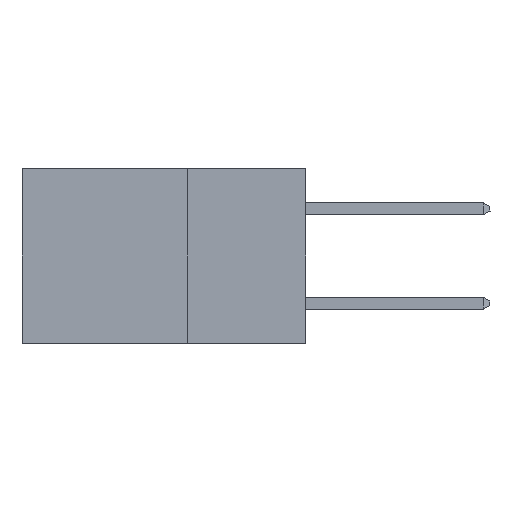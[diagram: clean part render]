
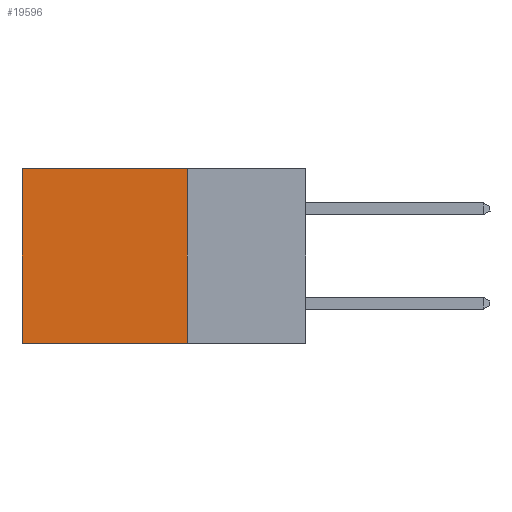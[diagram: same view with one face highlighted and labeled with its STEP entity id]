
A CAD part, left-side view. The second image highlights one B-rep face of the part: STEP entity #19596.
In plain terms, the highlighted planar face has unit normal (-1, 0, 0).
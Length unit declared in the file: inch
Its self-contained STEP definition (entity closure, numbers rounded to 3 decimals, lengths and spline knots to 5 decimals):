
#124 = VECTOR ( 'NONE', #10362, 39.37008 ) ;
#662 = EDGE_CURVE ( 'NONE', #23509, #13252, #12239, .T. ) ;
#1807 = CARTESIAN_POINT ( 'NONE',  ( 0.298, 0.25, -0.37 ) ) ;
#2325 = ORIENTED_EDGE ( 'NONE', *, *, #30814, .F. ) ;
#2909 = CARTESIAN_POINT ( 'NONE',  ( 0.298, 0.6, 0. ) ) ;
#3362 = CARTESIAN_POINT ( 'NONE',  ( 0.298, 0.25, 0. ) ) ;
#3587 = VERTEX_POINT ( 'NONE', #17950 ) ;
#3789 = DIRECTION ( 'NONE',  ( 0., 0., -1. ) ) ;
#4564 = DIRECTION ( 'NONE',  ( 0., 1., 0. ) ) ;
#4789 = DIRECTION ( 'NONE',  ( 0., 0., -1. ) ) ;
#5331 = ORIENTED_EDGE ( 'NONE', *, *, #23557, .T. ) ;
#5477 = VECTOR ( 'NONE', #4564, 39.37008 ) ;
#5871 = LINE ( 'NONE', #1807, #5477 ) ;
#7683 = DIRECTION ( 'NONE',  ( 0., 0., -1. ) ) ;
#7885 = LINE ( 'NONE', #2909, #26384 ) ;
#10362 = DIRECTION ( 'NONE',  ( 0., 1., 0. ) ) ;
#11005 = AXIS2_PLACEMENT_3D ( 'NONE', #16033, #16863, #4789 ) ;
#12239 = LINE ( 'NONE', #3362, #124 ) ;
#12748 = VECTOR ( 'NONE', #3789, 39.37008 ) ;
#13252 = VERTEX_POINT ( 'NONE', #20198 ) ;
#14552 = CARTESIAN_POINT ( 'NONE',  ( 0.298, 0.25, 0. ) ) ;
#15686 = EDGE_CURVE ( 'NONE', #23509, #3587, #18451, .T. ) ;
#16033 = CARTESIAN_POINT ( 'NONE',  ( 0.298, 0.25, 0. ) ) ;
#16215 = ORIENTED_EDGE ( 'NONE', *, *, #662, .T. ) ;
#16863 = DIRECTION ( 'NONE',  ( 1., 0., 0. ) ) ;
#17950 = CARTESIAN_POINT ( 'NONE',  ( 0.298, 0.25, -0.37 ) ) ;
#18451 = LINE ( 'NONE', #18626, #12748 ) ;
#18626 = CARTESIAN_POINT ( 'NONE',  ( 0.298, 0.25, 0. ) ) ;
#18630 = EDGE_LOOP ( 'NONE', ( #5331, #2325, #23736, #16215 ) ) ;
#19596 = ADVANCED_FACE ( 'NONE', ( #24249 ), #30500, .F. ) ;
#20198 = CARTESIAN_POINT ( 'NONE',  ( 0.298, 0.6, 0. ) ) ;
#20224 = VERTEX_POINT ( 'NONE', #26905 ) ;
#23509 = VERTEX_POINT ( 'NONE', #14552 ) ;
#23557 = EDGE_CURVE ( 'NONE', #13252, #20224, #7885, .T. ) ;
#23736 = ORIENTED_EDGE ( 'NONE', *, *, #15686, .F. ) ;
#24249 = FACE_OUTER_BOUND ( 'NONE', #18630, .T. ) ;
#26384 = VECTOR ( 'NONE', #7683, 39.37008 ) ;
#26905 = CARTESIAN_POINT ( 'NONE',  ( 0.298, 0.6, -0.37 ) ) ;
#30500 = PLANE ( 'NONE',  #11005 ) ;
#30814 = EDGE_CURVE ( 'NONE', #3587, #20224, #5871, .T. ) ;
